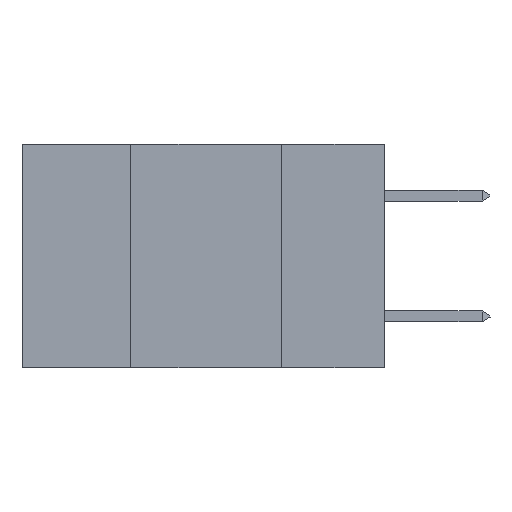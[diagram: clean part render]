
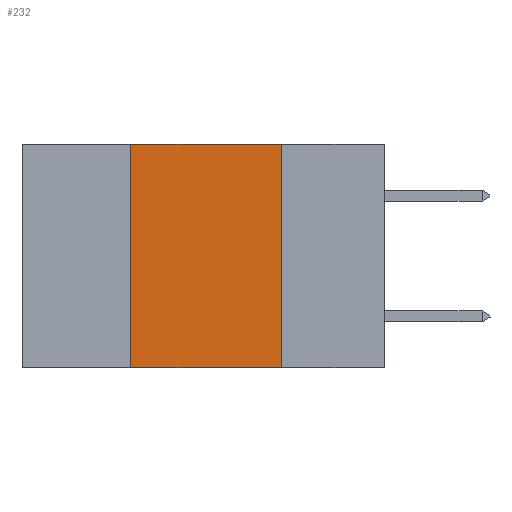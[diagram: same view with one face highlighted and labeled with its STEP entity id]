
A CAD part, left-side view. The second image highlights one B-rep face of the part: STEP entity #232.
In plain terms, the highlighted planar face has unit normal (-1, 0, 0).
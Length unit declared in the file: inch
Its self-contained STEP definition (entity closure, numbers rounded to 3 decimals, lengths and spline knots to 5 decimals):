
#232 = ADVANCED_FACE ( 'NONE', ( #13129 ), #9546, .F. ) ;
#259 = CARTESIAN_POINT ( 'NONE',  ( 0., 0.17, 0. ) ) ;
#1804 = VECTOR ( 'NONE', #12024, 39.37008 ) ;
#2416 = ORIENTED_EDGE ( 'NONE', *, *, #5108, .F. ) ;
#2577 = CARTESIAN_POINT ( 'NONE',  ( 0., 0.42, 0. ) ) ;
#3101 = AXIS2_PLACEMENT_3D ( 'NONE', #5225, #8932, #3965 ) ;
#3468 = EDGE_CURVE ( 'NONE', #6253, #12531, #8398, .T. ) ;
#3965 = DIRECTION ( 'NONE',  ( 0., 0., -1. ) ) ;
#4017 = ORIENTED_EDGE ( 'NONE', *, *, #5067, .F. ) ;
#4683 = VECTOR ( 'NONE', #12495, 39.37008 ) ;
#4854 = LINE ( 'NONE', #11965, #1804 ) ;
#4878 = EDGE_CURVE ( 'NONE', #9100, #8136, #7993, .T. ) ;
#5032 = CARTESIAN_POINT ( 'NONE',  ( 0., 0.17, -0.37 ) ) ;
#5067 = EDGE_CURVE ( 'NONE', #12531, #8136, #9233, .T. ) ;
#5108 = EDGE_CURVE ( 'NONE', #9100, #6253, #4854, .T. ) ;
#5225 = CARTESIAN_POINT ( 'NONE',  ( 0., 0.6, 0. ) ) ;
#5650 = DIRECTION ( 'NONE',  ( 0., -1., 0. ) ) ;
#5666 = CARTESIAN_POINT ( 'NONE',  ( 0., 0.6, 0. ) ) ;
#5847 = EDGE_LOOP ( 'NONE', ( #4017, #7319, #2416, #8749 ) ) ;
#6253 = VERTEX_POINT ( 'NONE', #2577 ) ;
#7319 = ORIENTED_EDGE ( 'NONE', *, *, #3468, .F. ) ;
#7993 = LINE ( 'NONE', #12496, #4683 ) ;
#8136 = VERTEX_POINT ( 'NONE', #5032 ) ;
#8398 = LINE ( 'NONE', #5666, #10564 ) ;
#8749 = ORIENTED_EDGE ( 'NONE', *, *, #4878, .T. ) ;
#8932 = DIRECTION ( 'NONE',  ( 1., 0., 0. ) ) ;
#9100 = VERTEX_POINT ( 'NONE', #10696 ) ;
#9233 = LINE ( 'NONE', #10993, #10956 ) ;
#9546 = PLANE ( 'NONE',  #3101 ) ;
#10564 = VECTOR ( 'NONE', #5650, 39.37008 ) ;
#10696 = CARTESIAN_POINT ( 'NONE',  ( 0., 0.42, -0.37 ) ) ;
#10892 = DIRECTION ( 'NONE',  ( 0., 0., -1. ) ) ;
#10956 = VECTOR ( 'NONE', #10892, 39.37008 ) ;
#10993 = CARTESIAN_POINT ( 'NONE',  ( 0., 0.17, 0. ) ) ;
#11965 = CARTESIAN_POINT ( 'NONE',  ( 0., 0.42, 0. ) ) ;
#12024 = DIRECTION ( 'NONE',  ( 0., 0., 1. ) ) ;
#12495 = DIRECTION ( 'NONE',  ( 0., -1., 0. ) ) ;
#12496 = CARTESIAN_POINT ( 'NONE',  ( 0., 0.6, -0.37 ) ) ;
#12531 = VERTEX_POINT ( 'NONE', #259 ) ;
#13129 = FACE_OUTER_BOUND ( 'NONE', #5847, .T. ) ;
